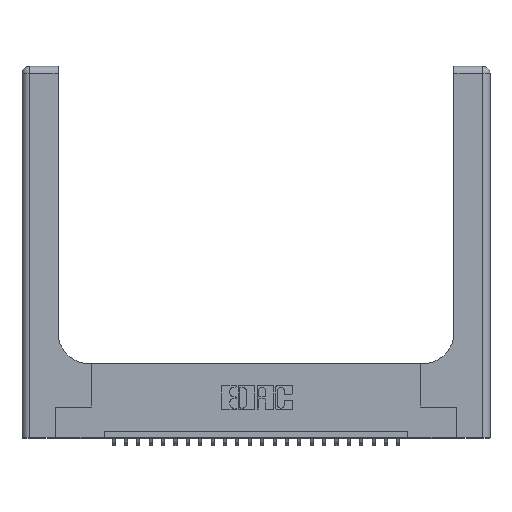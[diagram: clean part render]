
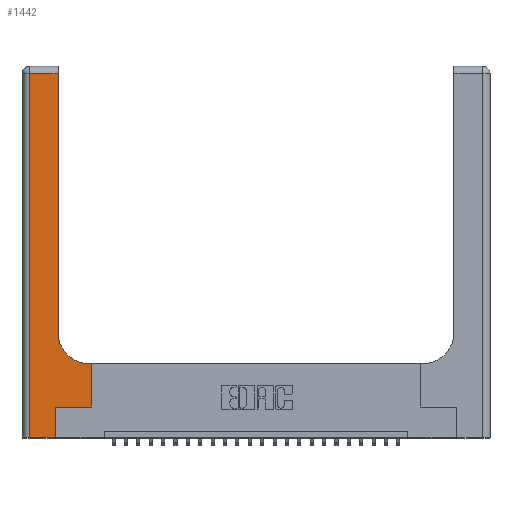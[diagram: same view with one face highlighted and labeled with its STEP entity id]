
A CAD part, top view. The second image highlights one B-rep face of the part: STEP entity #1442.
In plain terms, the highlighted planar face has unit normal (0, 0, 1).
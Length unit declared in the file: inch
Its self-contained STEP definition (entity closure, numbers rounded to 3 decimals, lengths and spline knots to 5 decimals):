
#1442 = ADVANCED_FACE ( 'NONE', ( #1455 ), #4987, .F. ) ;
#1455 = FACE_OUTER_BOUND ( 'NONE', #12086, .T. ) ;
#1689 = EDGE_CURVE ( 'NONE', #16859, #19167, #20102, .T. ) ;
#2178 = VECTOR ( 'NONE', #11758, 39.37008 ) ;
#2849 = DIRECTION ( 'NONE',  ( 1., 0., 0. ) ) ;
#3766 = DIRECTION ( 'NONE',  ( -1., 0., 0. ) ) ;
#3880 = VECTOR ( 'NONE', #22449, 39.37008 ) ;
#4539 = VECTOR ( 'NONE', #21106, 39.37008 ) ;
#4987 = PLANE ( 'NONE',  #10136 ) ;
#5428 = EDGE_CURVE ( 'NONE', #20635, #16859, #24320, .T. ) ;
#5692 = VERTEX_POINT ( 'NONE', #21372 ) ;
#6947 = CARTESIAN_POINT ( 'NONE',  ( 0.5415, 0.85, 0.37 ) ) ;
#6987 = CARTESIAN_POINT ( 'NONE',  ( 0., 3., 0.37 ) ) ;
#7066 = CARTESIAN_POINT ( 'NONE',  ( 0.06, 2.94, 0.37 ) ) ;
#7494 = LINE ( 'NONE', #17927, #2178 ) ;
#7503 = CARTESIAN_POINT ( 'NONE',  ( 0.269, 0., 0.37 ) ) ;
#7943 = CARTESIAN_POINT ( 'NONE',  ( 0.269, 0.25, 0.37 ) ) ;
#8414 = CARTESIAN_POINT ( 'NONE',  ( 0.269, 0.25, 0.37 ) ) ;
#8818 = VERTEX_POINT ( 'NONE', #11578 ) ;
#9620 = EDGE_CURVE ( 'NONE', #18247, #5692, #10124, .T. ) ;
#9769 = EDGE_CURVE ( 'NONE', #20023, #15515, #16614, .T. ) ;
#10124 = LINE ( 'NONE', #22368, #3880 ) ;
#10136 = AXIS2_PLACEMENT_3D ( 'NONE', #6987, #12950, #3766 ) ;
#10895 = CARTESIAN_POINT ( 'NONE',  ( 0., 0., 0.37 ) ) ;
#10930 = DIRECTION ( 'NONE',  ( 0., -1., 0. ) ) ;
#11578 = CARTESIAN_POINT ( 'NONE',  ( 0.06, 0., 0.37 ) ) ;
#11758 = DIRECTION ( 'NONE',  ( 0., 1., 0. ) ) ;
#12000 = ORIENTED_EDGE ( 'NONE', *, *, #1689, .T. ) ;
#12086 = EDGE_LOOP ( 'NONE', ( #21453, #12000, #13319, #24984, #19561, #24011, #19384, #18613, #17802 ) ) ;
#12818 = VECTOR ( 'NONE', #23387, 39.37008 ) ;
#12950 = DIRECTION ( 'NONE',  ( 0., 0., -1. ) ) ;
#13136 = AXIS2_PLACEMENT_3D ( 'NONE', #6947, #20664, #2849 ) ;
#13191 = VECTOR ( 'NONE', #10930, 39.37008 ) ;
#13319 = ORIENTED_EDGE ( 'NONE', *, *, #24146, .T. ) ;
#13556 = CARTESIAN_POINT ( 'NONE',  ( 0., 2.94, 0.37 ) ) ;
#13946 = CARTESIAN_POINT ( 'NONE',  ( 0.2915, 2.94, 0.37 ) ) ;
#15336 = EDGE_CURVE ( 'NONE', #8818, #22339, #22613, .T. ) ;
#15515 = VERTEX_POINT ( 'NONE', #15648 ) ;
#15648 = CARTESIAN_POINT ( 'NONE',  ( 0.5585, 0.25, 0.37 ) ) ;
#15802 = EDGE_CURVE ( 'NONE', #5692, #20635, #25373, .T. ) ;
#16190 = CARTESIAN_POINT ( 'NONE',  ( 0.269, 0., 0.37 ) ) ;
#16412 = DIRECTION ( 'NONE',  ( 1., 0., 0. ) ) ;
#16614 = LINE ( 'NONE', #8414, #21296 ) ;
#16859 = VERTEX_POINT ( 'NONE', #13946 ) ;
#17572 = CARTESIAN_POINT ( 'NONE',  ( 0.2915, 3., 0.37 ) ) ;
#17802 = ORIENTED_EDGE ( 'NONE', *, *, #15802, .T. ) ;
#17927 = CARTESIAN_POINT ( 'NONE',  ( 0.5585, 0.25, 0.37 ) ) ;
#18002 = CARTESIAN_POINT ( 'NONE',  ( 0.2915, 0.85, 0.37 ) ) ;
#18247 = VERTEX_POINT ( 'NONE', #22076 ) ;
#18613 = ORIENTED_EDGE ( 'NONE', *, *, #9620, .T. ) ;
#19167 = VERTEX_POINT ( 'NONE', #7066 ) ;
#19361 = EDGE_CURVE ( 'NONE', #15515, #18247, #7494, .T. ) ;
#19384 = ORIENTED_EDGE ( 'NONE', *, *, #19361, .T. ) ;
#19561 = ORIENTED_EDGE ( 'NONE', *, *, #22004, .T. ) ;
#20023 = VERTEX_POINT ( 'NONE', #7943 ) ;
#20102 = LINE ( 'NONE', #13556, #4539 ) ;
#20148 = LINE ( 'NONE', #16190, #21060 ) ;
#20635 = VERTEX_POINT ( 'NONE', #18002 ) ;
#20664 = DIRECTION ( 'NONE',  ( 0., 0., -1. ) ) ;
#21060 = VECTOR ( 'NONE', #24090, 39.37008 ) ;
#21106 = DIRECTION ( 'NONE',  ( -1., 0., 0. ) ) ;
#21296 = VECTOR ( 'NONE', #16412, 39.37008 ) ;
#21372 = CARTESIAN_POINT ( 'NONE',  ( 0.5415, 0.6, 0.37 ) ) ;
#21453 = ORIENTED_EDGE ( 'NONE', *, *, #5428, .T. ) ;
#22004 = EDGE_CURVE ( 'NONE', #22339, #20023, #20148, .T. ) ;
#22076 = CARTESIAN_POINT ( 'NONE',  ( 0.5585, 0.6, 0.37 ) ) ;
#22309 = VECTOR ( 'NONE', #24765, 39.37008 ) ;
#22339 = VERTEX_POINT ( 'NONE', #7503 ) ;
#22368 = CARTESIAN_POINT ( 'NONE',  ( 0.2915, 0.6, 0.37 ) ) ;
#22449 = DIRECTION ( 'NONE',  ( -1., 0., 0. ) ) ;
#22613 = LINE ( 'NONE', #10895, #22309 ) ;
#22829 = CARTESIAN_POINT ( 'NONE',  ( 0.06, 3., 0.37 ) ) ;
#23387 = DIRECTION ( 'NONE',  ( 0., 1., 0. ) ) ;
#24011 = ORIENTED_EDGE ( 'NONE', *, *, #9769, .T. ) ;
#24090 = DIRECTION ( 'NONE',  ( 0., 1., 0. ) ) ;
#24146 = EDGE_CURVE ( 'NONE', #19167, #8818, #25642, .T. ) ;
#24320 = LINE ( 'NONE', #17572, #12818 ) ;
#24765 = DIRECTION ( 'NONE',  ( 1., 0., 0. ) ) ;
#24984 = ORIENTED_EDGE ( 'NONE', *, *, #15336, .T. ) ;
#25373 = CIRCLE ( 'NONE', #13136, 0.25 ) ;
#25642 = LINE ( 'NONE', #22829, #13191 ) ;
